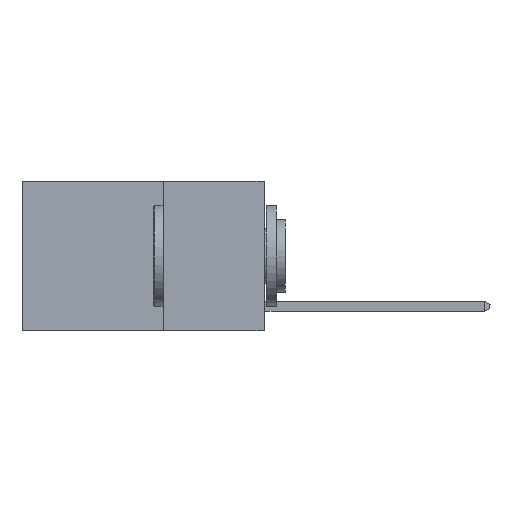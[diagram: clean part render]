
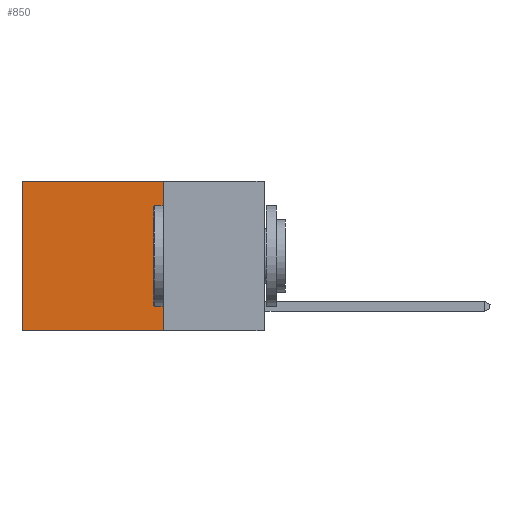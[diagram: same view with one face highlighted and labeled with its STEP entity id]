
A CAD part, left-side view. The second image highlights one B-rep face of the part: STEP entity #850.
In plain terms, the highlighted planar face has unit normal (-1, 0, 0).
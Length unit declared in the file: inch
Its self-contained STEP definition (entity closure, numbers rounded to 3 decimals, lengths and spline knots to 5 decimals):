
#160 = CARTESIAN_POINT ( 'NONE',  ( 0.2625, 0.25, -0.37 ) ) ;
#383 = FACE_OUTER_BOUND ( 'NONE', #15543, .T. ) ;
#850 = ADVANCED_FACE ( 'NONE', ( #383 ), #6088, .F. ) ;
#1315 = DIRECTION ( 'NONE',  ( 0., 0., -1. ) ) ;
#1500 = VERTEX_POINT ( 'NONE', #160 ) ;
#1515 = ORIENTED_EDGE ( 'NONE', *, *, #15224, .T. ) ;
#2037 = DIRECTION ( 'NONE',  ( 0., 0., -1. ) ) ;
#2304 = DIRECTION ( 'NONE',  ( 0., 0., -1. ) ) ;
#2849 = VERTEX_POINT ( 'NONE', #11141 ) ;
#2911 = EDGE_CURVE ( 'NONE', #12999, #1500, #5331, .T. ) ;
#3870 = ORIENTED_EDGE ( 'NONE', *, *, #2911, .F. ) ;
#3990 = VECTOR ( 'NONE', #2037, 39.37008 ) ;
#4096 = DIRECTION ( 'NONE',  ( 0., 1., 0. ) ) ;
#4379 = LINE ( 'NONE', #4855, #6615 ) ;
#4670 = DIRECTION ( 'NONE',  ( 1., 0., 0. ) ) ;
#4855 = CARTESIAN_POINT ( 'NONE',  ( 0.2625, 0.25, -0.37 ) ) ;
#5139 = AXIS2_PLACEMENT_3D ( 'NONE', #10004, #4670, #2304 ) ;
#5331 = LINE ( 'NONE', #15292, #9481 ) ;
#6088 = PLANE ( 'NONE',  #5139 ) ;
#6286 = DIRECTION ( 'NONE',  ( 0., 1., 0. ) ) ;
#6615 = VECTOR ( 'NONE', #6286, 39.37008 ) ;
#6753 = EDGE_CURVE ( 'NONE', #9848, #2849, #14537, .T. ) ;
#7276 = ORIENTED_EDGE ( 'NONE', *, *, #15949, .F. ) ;
#7319 = CARTESIAN_POINT ( 'NONE',  ( 0.2625, 0.25, 0. ) ) ;
#7350 = CARTESIAN_POINT ( 'NONE',  ( 0.2625, 0.25, 0. ) ) ;
#7951 = LINE ( 'NONE', #7319, #11108 ) ;
#9481 = VECTOR ( 'NONE', #1315, 39.37008 ) ;
#9848 = VERTEX_POINT ( 'NONE', #10535 ) ;
#10004 = CARTESIAN_POINT ( 'NONE',  ( 0.2625, 0.25, 0. ) ) ;
#10535 = CARTESIAN_POINT ( 'NONE',  ( 0.2625, 0.6, 0. ) ) ;
#11108 = VECTOR ( 'NONE', #4096, 39.37008 ) ;
#11141 = CARTESIAN_POINT ( 'NONE',  ( 0.2625, 0.6, -0.37 ) ) ;
#12999 = VERTEX_POINT ( 'NONE', #7350 ) ;
#13664 = ORIENTED_EDGE ( 'NONE', *, *, #6753, .T. ) ;
#14537 = LINE ( 'NONE', #16047, #3990 ) ;
#15224 = EDGE_CURVE ( 'NONE', #12999, #9848, #7951, .T. ) ;
#15292 = CARTESIAN_POINT ( 'NONE',  ( 0.2625, 0.25, 0. ) ) ;
#15543 = EDGE_LOOP ( 'NONE', ( #13664, #7276, #3870, #1515 ) ) ;
#15949 = EDGE_CURVE ( 'NONE', #1500, #2849, #4379, .T. ) ;
#16047 = CARTESIAN_POINT ( 'NONE',  ( 0.2625, 0.6, 0. ) ) ;
